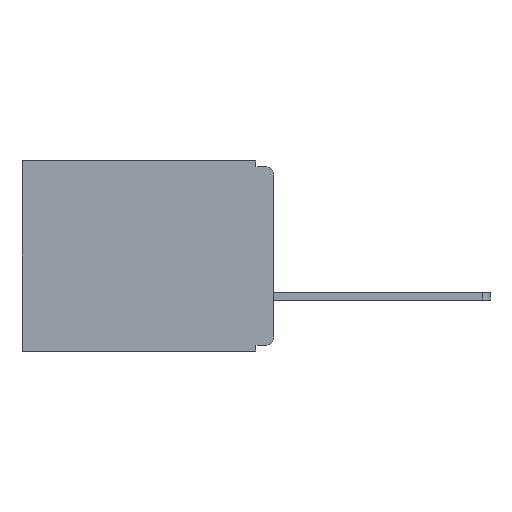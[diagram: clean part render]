
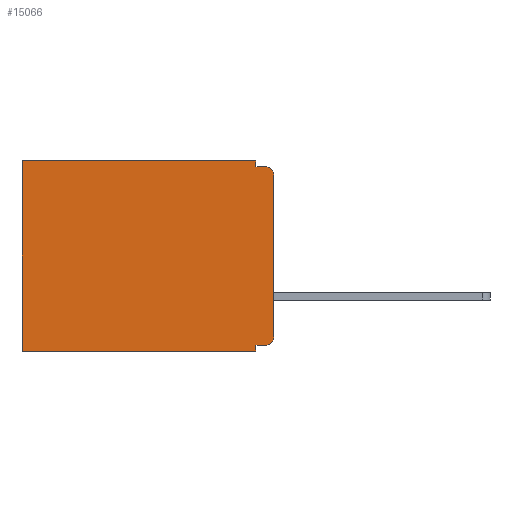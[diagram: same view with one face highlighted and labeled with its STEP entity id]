
A CAD part, left-side view. The second image highlights one B-rep face of the part: STEP entity #15066.
In plain terms, the highlighted planar face has unit normal (-1, 0, 0).
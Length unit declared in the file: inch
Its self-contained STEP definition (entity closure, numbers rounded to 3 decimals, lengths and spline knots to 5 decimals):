
#114 = VECTOR ( 'NONE', #9383, 39.37008 ) ;
#871 = DIRECTION ( 'NONE',  ( -1., 0., 0. ) ) ;
#1257 = CIRCLE ( 'NONE', #9087, 0.015 ) ;
#1271 = CARTESIAN_POINT ( 'NONE',  ( 0.3, 0.031, -0.33 ) ) ;
#1642 = VERTEX_POINT ( 'NONE', #15428 ) ;
#1844 = LINE ( 'NONE', #16947, #6876 ) ;
#2298 = ORIENTED_EDGE ( 'NONE', *, *, #23122, .F. ) ;
#2483 = VECTOR ( 'NONE', #15296, 39.37008 ) ;
#3150 = VECTOR ( 'NONE', #16381, 39.37008 ) ;
#3156 = ORIENTED_EDGE ( 'NONE', *, *, #10513, .T. ) ;
#3498 = DIRECTION ( 'NONE',  ( 1., 0., 0. ) ) ;
#3977 = CARTESIAN_POINT ( 'NONE',  ( 0.3, 0.031, -0.33 ) ) ;
#4002 = DIRECTION ( 'NONE',  ( 0., 0., -1. ) ) ;
#4074 = EDGE_CURVE ( 'NONE', #1642, #24937, #1257, .T. ) ;
#4570 = LINE ( 'NONE', #16676, #5235 ) ;
#5235 = VECTOR ( 'NONE', #4002, 39.37008 ) ;
#5448 = EDGE_CURVE ( 'NONE', #19373, #7014, #1844, .T. ) ;
#5647 = ORIENTED_EDGE ( 'NONE', *, *, #6105, .T. ) ;
#6037 = CARTESIAN_POINT ( 'NONE',  ( 0.3, 0.015, -0.025 ) ) ;
#6105 = EDGE_CURVE ( 'NONE', #17470, #7014, #6543, .T. ) ;
#6466 = LINE ( 'NONE', #13607, #114 ) ;
#6507 = ORIENTED_EDGE ( 'NONE', *, *, #17427, .T. ) ;
#6543 = LINE ( 'NONE', #27251, #22673 ) ;
#6876 = VECTOR ( 'NONE', #17486, 39.37008 ) ;
#7014 = VERTEX_POINT ( 'NONE', #8673 ) ;
#7920 = ORIENTED_EDGE ( 'NONE', *, *, #4074, .T. ) ;
#8224 = DIRECTION ( 'NONE',  ( 0., 0., -1. ) ) ;
#8673 = CARTESIAN_POINT ( 'NONE',  ( 0.3, 0.437, -0.33 ) ) ;
#9087 = AXIS2_PLACEMENT_3D ( 'NONE', #27198, #871, #10130 ) ;
#9383 = DIRECTION ( 'NONE',  ( 0., -1., 0. ) ) ;
#9436 = AXIS2_PLACEMENT_3D ( 'NONE', #6037, #20807, #8224 ) ;
#9644 = VECTOR ( 'NONE', #15163, 39.37008 ) ;
#10036 = VECTOR ( 'NONE', #24532, 39.37008 ) ;
#10130 = DIRECTION ( 'NONE',  ( 0., 0., -1. ) ) ;
#10399 = EDGE_LOOP ( 'NONE', ( #11608, #6507, #13118, #2298, #3156, #5647, #13546, #22864, #18524, #7920 ) ) ;
#10446 = CARTESIAN_POINT ( 'NONE',  ( 0.3, 0., -0.025 ) ) ;
#10513 = EDGE_CURVE ( 'NONE', #24524, #17470, #11615, .T. ) ;
#11162 = VERTEX_POINT ( 'NONE', #10446 ) ;
#11608 = ORIENTED_EDGE ( 'NONE', *, *, #13038, .F. ) ;
#11615 = LINE ( 'NONE', #19312, #9644 ) ;
#11740 = CARTESIAN_POINT ( 'NONE',  ( 0.3, 0.031, -0.01 ) ) ;
#12546 = CARTESIAN_POINT ( 'NONE',  ( 0.3, 0.437, 0. ) ) ;
#12761 = AXIS2_PLACEMENT_3D ( 'NONE', #14084, #3498, #18298 ) ;
#13038 = EDGE_CURVE ( 'NONE', #11162, #24937, #4570, .T. ) ;
#13118 = ORIENTED_EDGE ( 'NONE', *, *, #17821, .F. ) ;
#13469 = CARTESIAN_POINT ( 'NONE',  ( 0.3, 0., -0.305 ) ) ;
#13546 = ORIENTED_EDGE ( 'NONE', *, *, #5448, .F. ) ;
#13607 = CARTESIAN_POINT ( 'NONE',  ( 0.3, 0., -0.01 ) ) ;
#14073 = FACE_OUTER_BOUND ( 'NONE', #10399, .T. ) ;
#14084 = CARTESIAN_POINT ( 'NONE',  ( 0.3, 0., -0.33 ) ) ;
#14300 = CARTESIAN_POINT ( 'NONE',  ( 0.3, 0., -0.32 ) ) ;
#15066 = ADVANCED_FACE ( 'NONE', ( #14073 ), #26567, .F. ) ;
#15163 = DIRECTION ( 'NONE',  ( 0., 1., 0. ) ) ;
#15296 = DIRECTION ( 'NONE',  ( 0., 0., -1. ) ) ;
#15428 = CARTESIAN_POINT ( 'NONE',  ( 0.3, 0.015, -0.32 ) ) ;
#15869 = CARTESIAN_POINT ( 'NONE',  ( 0.3, 0.031, 0. ) ) ;
#16381 = DIRECTION ( 'NONE',  ( 0., 1., 0. ) ) ;
#16676 = CARTESIAN_POINT ( 'NONE',  ( 0.3, 0., -0.33 ) ) ;
#16947 = CARTESIAN_POINT ( 'NONE',  ( 0.3, 0., -0.33 ) ) ;
#17190 = DIRECTION ( 'NONE',  ( 0., 0., -1. ) ) ;
#17427 = EDGE_CURVE ( 'NONE', #11162, #24303, #20528, .T. ) ;
#17470 = VERTEX_POINT ( 'NONE', #12546 ) ;
#17486 = DIRECTION ( 'NONE',  ( 0., 1., 0. ) ) ;
#17821 = EDGE_CURVE ( 'NONE', #22031, #24303, #6466, .T. ) ;
#18298 = DIRECTION ( 'NONE',  ( 0., 0., -1. ) ) ;
#18524 = ORIENTED_EDGE ( 'NONE', *, *, #26304, .F. ) ;
#19191 = EDGE_CURVE ( 'NONE', #22681, #19373, #21226, .T. ) ;
#19312 = CARTESIAN_POINT ( 'NONE',  ( 0.3, 0., 0. ) ) ;
#19373 = VERTEX_POINT ( 'NONE', #3977 ) ;
#20043 = LINE ( 'NONE', #14300, #3150 ) ;
#20528 = CIRCLE ( 'NONE', #9436, 0.015 ) ;
#20807 = DIRECTION ( 'NONE',  ( -1., 0., 0. ) ) ;
#21226 = LINE ( 'NONE', #1271, #10036 ) ;
#21411 = CARTESIAN_POINT ( 'NONE',  ( 0.3, 0.015, -0.01 ) ) ;
#22031 = VERTEX_POINT ( 'NONE', #11740 ) ;
#22673 = VECTOR ( 'NONE', #17190, 39.37008 ) ;
#22681 = VERTEX_POINT ( 'NONE', #24222 ) ;
#22864 = ORIENTED_EDGE ( 'NONE', *, *, #19191, .F. ) ;
#23122 = EDGE_CURVE ( 'NONE', #24524, #22031, #24284, .T. ) ;
#24222 = CARTESIAN_POINT ( 'NONE',  ( 0.3, 0.031, -0.32 ) ) ;
#24284 = LINE ( 'NONE', #25719, #2483 ) ;
#24303 = VERTEX_POINT ( 'NONE', #21411 ) ;
#24524 = VERTEX_POINT ( 'NONE', #15869 ) ;
#24532 = DIRECTION ( 'NONE',  ( 0., 0., -1. ) ) ;
#24937 = VERTEX_POINT ( 'NONE', #13469 ) ;
#25719 = CARTESIAN_POINT ( 'NONE',  ( 0.3, 0.031, 0. ) ) ;
#26304 = EDGE_CURVE ( 'NONE', #1642, #22681, #20043, .T. ) ;
#26567 = PLANE ( 'NONE',  #12761 ) ;
#27198 = CARTESIAN_POINT ( 'NONE',  ( 0.3, 0.015, -0.305 ) ) ;
#27251 = CARTESIAN_POINT ( 'NONE',  ( 0.3, 0.437, -0.33 ) ) ;
